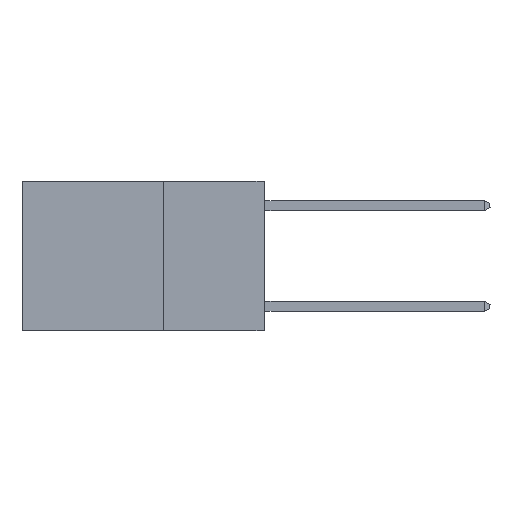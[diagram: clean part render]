
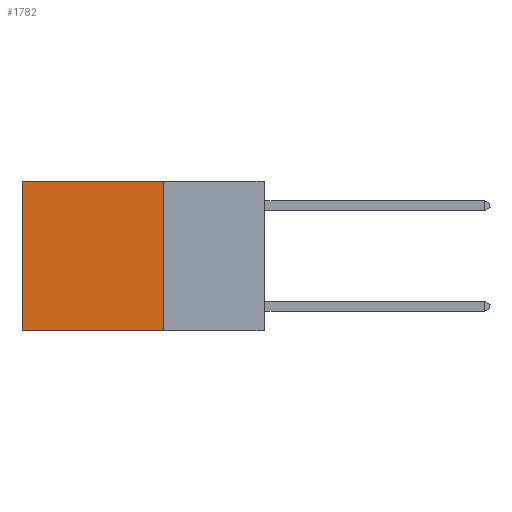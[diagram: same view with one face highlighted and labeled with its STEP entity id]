
A CAD part, left-side view. The second image highlights one B-rep face of the part: STEP entity #1782.
In plain terms, the highlighted planar face has unit normal (-1, 0, 0).
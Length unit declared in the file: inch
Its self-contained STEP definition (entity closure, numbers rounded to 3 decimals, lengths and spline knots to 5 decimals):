
#7 = DIRECTION ( 'NONE',  ( 0., 0., -1. ) ) ;
#65 = VERTEX_POINT ( 'NONE', #12796 ) ;
#88 = CARTESIAN_POINT ( 'NONE',  ( 0.2625, 0.25, 0. ) ) ;
#633 = DIRECTION ( 'NONE',  ( 0., 0., -1. ) ) ;
#1087 = CARTESIAN_POINT ( 'NONE',  ( 0.2625, 0.25, -0.37 ) ) ;
#1582 = CARTESIAN_POINT ( 'NONE',  ( 0.2625, 0.25, 0. ) ) ;
#1782 = ADVANCED_FACE ( 'NONE', ( #5468 ), #15398, .F. ) ;
#2451 = VERTEX_POINT ( 'NONE', #7298 ) ;
#3135 = LINE ( 'NONE', #11425, #4472 ) ;
#3812 = VERTEX_POINT ( 'NONE', #1087 ) ;
#3945 = DIRECTION ( 'NONE',  ( 0., 1., 0. ) ) ;
#4472 = VECTOR ( 'NONE', #8105, 39.37008 ) ;
#4520 = AXIS2_PLACEMENT_3D ( 'NONE', #1582, #10276, #5226 ) ;
#5226 = DIRECTION ( 'NONE',  ( 0., 0., -1. ) ) ;
#5468 = FACE_OUTER_BOUND ( 'NONE', #14190, .T. ) ;
#5816 = VERTEX_POINT ( 'NONE', #8359 ) ;
#6358 = LINE ( 'NONE', #11310, #14720 ) ;
#7298 = CARTESIAN_POINT ( 'NONE',  ( 0.2625, 0.6, -0.37 ) ) ;
#8008 = VECTOR ( 'NONE', #633, 39.37008 ) ;
#8105 = DIRECTION ( 'NONE',  ( 0., 1., 0. ) ) ;
#8359 = CARTESIAN_POINT ( 'NONE',  ( 0.2625, 0.6, 0. ) ) ;
#8826 = EDGE_CURVE ( 'NONE', #65, #5816, #3135, .T. ) ;
#9009 = ORIENTED_EDGE ( 'NONE', *, *, #9179, .F. ) ;
#9058 = EDGE_CURVE ( 'NONE', #65, #3812, #11237, .T. ) ;
#9179 = EDGE_CURVE ( 'NONE', #3812, #2451, #6358, .T. ) ;
#9192 = LINE ( 'NONE', #12014, #8008 ) ;
#10276 = DIRECTION ( 'NONE',  ( 1., 0., 0. ) ) ;
#10306 = VECTOR ( 'NONE', #7, 39.37008 ) ;
#10778 = ORIENTED_EDGE ( 'NONE', *, *, #9058, .F. ) ;
#11237 = LINE ( 'NONE', #88, #10306 ) ;
#11310 = CARTESIAN_POINT ( 'NONE',  ( 0.2625, 0.25, -0.37 ) ) ;
#11425 = CARTESIAN_POINT ( 'NONE',  ( 0.2625, 0.25, 0. ) ) ;
#12014 = CARTESIAN_POINT ( 'NONE',  ( 0.2625, 0.6, 0. ) ) ;
#12796 = CARTESIAN_POINT ( 'NONE',  ( 0.2625, 0.25, 0. ) ) ;
#14190 = EDGE_LOOP ( 'NONE', ( #14913, #9009, #10778, #15248 ) ) ;
#14648 = EDGE_CURVE ( 'NONE', #5816, #2451, #9192, .T. ) ;
#14720 = VECTOR ( 'NONE', #3945, 39.37008 ) ;
#14913 = ORIENTED_EDGE ( 'NONE', *, *, #14648, .T. ) ;
#15248 = ORIENTED_EDGE ( 'NONE', *, *, #8826, .T. ) ;
#15398 = PLANE ( 'NONE',  #4520 ) ;
